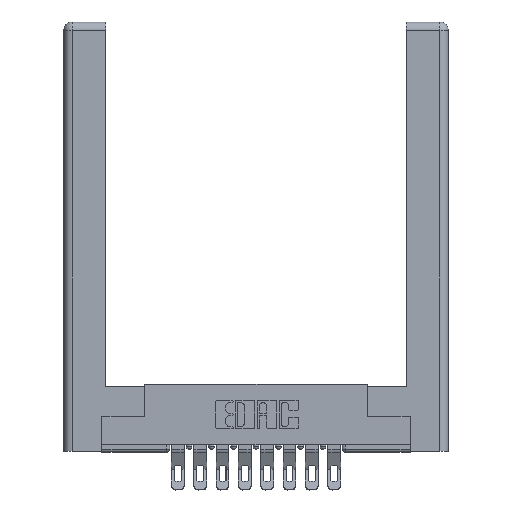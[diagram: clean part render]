
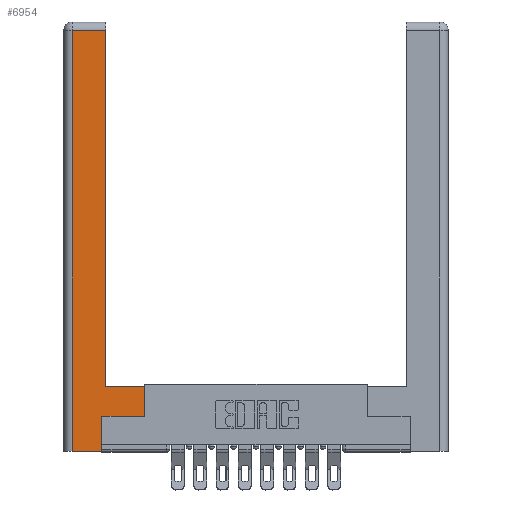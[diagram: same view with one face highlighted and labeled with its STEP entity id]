
A CAD part, top view. The second image highlights one B-rep face of the part: STEP entity #6954.
In plain terms, the highlighted planar face has unit normal (0, 0, 1).
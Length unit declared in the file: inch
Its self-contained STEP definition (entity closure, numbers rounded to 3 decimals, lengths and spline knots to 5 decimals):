
#496 = ORIENTED_EDGE ( 'NONE', *, *, #1650, .T. ) ;
#797 = CARTESIAN_POINT ( 'NONE',  ( 0.0615, 2.94, 0. ) ) ;
#882 = FACE_OUTER_BOUND ( 'NONE', #6579, .T. ) ;
#1161 = LINE ( 'NONE', #7992, #1297 ) ;
#1205 = LINE ( 'NONE', #1953, #2353 ) ;
#1297 = VECTOR ( 'NONE', #11084, 39.37008 ) ;
#1300 = DIRECTION ( 'NONE',  ( -1., 0., 0. ) ) ;
#1408 = DIRECTION ( 'NONE',  ( 0., 1., 0. ) ) ;
#1650 = EDGE_CURVE ( 'NONE', #8880, #7066, #14304, .T. ) ;
#1687 = VECTOR ( 'NONE', #8484, 39.37008 ) ;
#1953 = CARTESIAN_POINT ( 'NONE',  ( 0.265, 0.245, 0. ) ) ;
#2114 = EDGE_CURVE ( 'NONE', #9379, #8490, #1205, .T. ) ;
#2353 = VECTOR ( 'NONE', #7605, 39.37008 ) ;
#2487 = EDGE_CURVE ( 'NONE', #7261, #8230, #8699, .T. ) ;
#2836 = LINE ( 'NONE', #7307, #7276 ) ;
#3709 = CARTESIAN_POINT ( 'NONE',  ( 0.565, 0.245, 0. ) ) ;
#3731 = CARTESIAN_POINT ( 'NONE',  ( 0.565, 0.45, 0. ) ) ;
#3968 = CARTESIAN_POINT ( 'NONE',  ( 0.565, 0.45, 0. ) ) ;
#4000 = CARTESIAN_POINT ( 'NONE',  ( 0.0615, 0., 0. ) ) ;
#4510 = DIRECTION ( 'NONE',  ( 1., 0., 0. ) ) ;
#4894 = VECTOR ( 'NONE', #13280, 39.37008 ) ;
#4907 = CARTESIAN_POINT ( 'NONE',  ( 0.295, 0.45, 0. ) ) ;
#6157 = ORIENTED_EDGE ( 'NONE', *, *, #10373, .T. ) ;
#6170 = CARTESIAN_POINT ( 'NONE',  ( 0.265, 0., 0. ) ) ;
#6274 = LINE ( 'NONE', #8437, #8343 ) ;
#6373 = DIRECTION ( 'NONE',  ( 0., 0., -1. ) ) ;
#6397 = VECTOR ( 'NONE', #1300, 39.37008 ) ;
#6579 = EDGE_LOOP ( 'NONE', ( #11495, #496, #12920, #6851, #9291, #6157, #12545, #13690 ) ) ;
#6773 = EDGE_CURVE ( 'NONE', #7362, #8880, #6822, .T. ) ;
#6809 = CARTESIAN_POINT ( 'NONE',  ( 0.265, 0.245, 0. ) ) ;
#6822 = LINE ( 'NONE', #11470, #7610 ) ;
#6851 = ORIENTED_EDGE ( 'NONE', *, *, #7529, .T. ) ;
#6954 = ADVANCED_FACE ( 'NONE', ( #882 ), #14233, .F. ) ;
#7050 = AXIS2_PLACEMENT_3D ( 'NONE', #11899, #6373, #8683 ) ;
#7066 = VERTEX_POINT ( 'NONE', #7483 ) ;
#7261 = VERTEX_POINT ( 'NONE', #3709 ) ;
#7276 = VECTOR ( 'NONE', #4510, 39.37008 ) ;
#7307 = CARTESIAN_POINT ( 'NONE',  ( 0.265, 0., 0. ) ) ;
#7362 = VERTEX_POINT ( 'NONE', #4907 ) ;
#7483 = CARTESIAN_POINT ( 'NONE',  ( 0.0615, 2.94, 0. ) ) ;
#7529 = EDGE_CURVE ( 'NONE', #10637, #9379, #2836, .T. ) ;
#7605 = DIRECTION ( 'NONE',  ( 0., 1., 0. ) ) ;
#7610 = VECTOR ( 'NONE', #1408, 39.37008 ) ;
#7992 = CARTESIAN_POINT ( 'NONE',  ( 0.565, 0.245, 0. ) ) ;
#8051 = CARTESIAN_POINT ( 'NONE',  ( 0.295, 0.45, 0. ) ) ;
#8230 = VERTEX_POINT ( 'NONE', #3731 ) ;
#8343 = VECTOR ( 'NONE', #12903, 39.37008 ) ;
#8437 = CARTESIAN_POINT ( 'NONE',  ( 0.0615, 0., 0. ) ) ;
#8484 = DIRECTION ( 'NONE',  ( 0., 1., 0. ) ) ;
#8490 = VERTEX_POINT ( 'NONE', #6809 ) ;
#8683 = DIRECTION ( 'NONE',  ( -1., 0., 0. ) ) ;
#8699 = LINE ( 'NONE', #3968, #1687 ) ;
#8880 = VERTEX_POINT ( 'NONE', #14079 ) ;
#8947 = EDGE_CURVE ( 'NONE', #8230, #7362, #11226, .T. ) ;
#9291 = ORIENTED_EDGE ( 'NONE', *, *, #2114, .T. ) ;
#9379 = VERTEX_POINT ( 'NONE', #6170 ) ;
#10373 = EDGE_CURVE ( 'NONE', #8490, #7261, #1161, .T. ) ;
#10563 = EDGE_CURVE ( 'NONE', #7066, #10637, #6274, .T. ) ;
#10637 = VERTEX_POINT ( 'NONE', #4000 ) ;
#11084 = DIRECTION ( 'NONE',  ( 1., 0., 0. ) ) ;
#11226 = LINE ( 'NONE', #8051, #6397 ) ;
#11470 = CARTESIAN_POINT ( 'NONE',  ( 0.295, 3., 0. ) ) ;
#11495 = ORIENTED_EDGE ( 'NONE', *, *, #6773, .T. ) ;
#11899 = CARTESIAN_POINT ( 'NONE',  ( 0., 0., 0. ) ) ;
#12545 = ORIENTED_EDGE ( 'NONE', *, *, #2487, .T. ) ;
#12903 = DIRECTION ( 'NONE',  ( 0., -1., 0. ) ) ;
#12920 = ORIENTED_EDGE ( 'NONE', *, *, #10563, .T. ) ;
#13280 = DIRECTION ( 'NONE',  ( -1., 0., 0. ) ) ;
#13690 = ORIENTED_EDGE ( 'NONE', *, *, #8947, .T. ) ;
#14079 = CARTESIAN_POINT ( 'NONE',  ( 0.295, 2.94, 0. ) ) ;
#14233 = PLANE ( 'NONE',  #7050 ) ;
#14304 = LINE ( 'NONE', #797, #4894 ) ;
